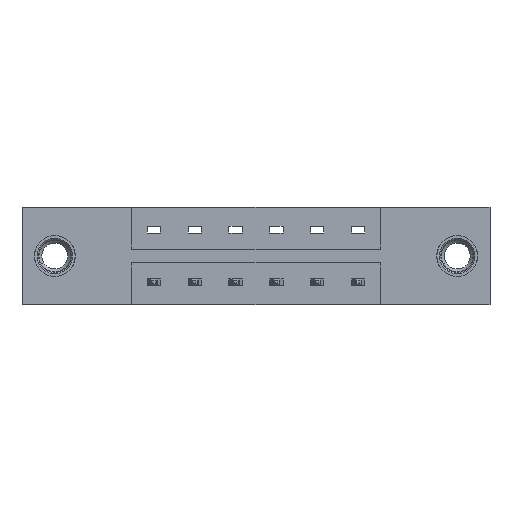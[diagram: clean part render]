
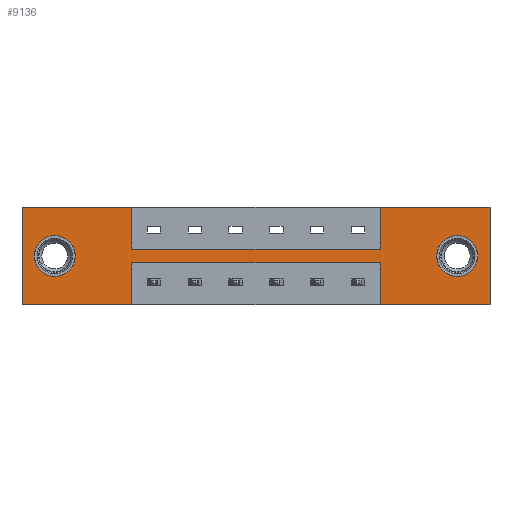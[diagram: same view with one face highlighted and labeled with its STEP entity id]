
A CAD part, front view. The second image highlights one B-rep face of the part: STEP entity #9136.
In plain terms, the highlighted planar face has unit normal (0, -1, 0).
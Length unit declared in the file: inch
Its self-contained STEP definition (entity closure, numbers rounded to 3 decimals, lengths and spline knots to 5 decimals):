
#42 = EDGE_CURVE ( 'NONE', #6262, #1896, #3276, .T. ) ;
#59 = CARTESIAN_POINT ( 'NONE',  ( 0.125, 0., -0.185 ) ) ;
#103 = DIRECTION ( 'NONE',  ( 0., 0., -1. ) ) ;
#153 = CARTESIAN_POINT ( 'NONE',  ( 0.4175, 0., -0.2115 ) ) ;
#176 = VECTOR ( 'NONE', #2613, 39.37008 ) ;
#224 = CIRCLE ( 'NONE', #9170, 0.078 ) ;
#268 = ORIENTED_EDGE ( 'NONE', *, *, #4116, .F. ) ;
#306 = EDGE_CURVE ( 'NONE', #5752, #7579, #224, .T. ) ;
#448 = EDGE_CURVE ( 'NONE', #5555, #4148, #8287, .T. ) ;
#486 = EDGE_CURVE ( 'NONE', #7261, #4726, #8028, .T. ) ;
#496 = CARTESIAN_POINT ( 'NONE',  ( 1.784, 0., -0.37 ) ) ;
#527 = VECTOR ( 'NONE', #1350, 39.37008 ) ;
#580 = EDGE_CURVE ( 'NONE', #7845, #5018, #1256, .T. ) ;
#640 = ORIENTED_EDGE ( 'NONE', *, *, #42, .F. ) ;
#680 = CARTESIAN_POINT ( 'NONE',  ( 0.125, 0., -0.107 ) ) ;
#698 = ORIENTED_EDGE ( 'NONE', *, *, #8571, .T. ) ;
#761 = DIRECTION ( 'NONE',  ( 0., 0., 1. ) ) ;
#824 = CARTESIAN_POINT ( 'NONE',  ( 0.4175, 0., -0.37 ) ) ;
#830 = ORIENTED_EDGE ( 'NONE', *, *, #5171, .T. ) ;
#857 = CARTESIAN_POINT ( 'NONE',  ( 0., 0., -0.37 ) ) ;
#1021 = LINE ( 'NONE', #7696, #5488 ) ;
#1100 = VERTEX_POINT ( 'NONE', #4235 ) ;
#1187 = ORIENTED_EDGE ( 'NONE', *, *, #1646, .F. ) ;
#1199 = FACE_BOUND ( 'NONE', #2375, .T. ) ;
#1221 = AXIS2_PLACEMENT_3D ( 'NONE', #6427, #3348, #5008 ) ;
#1256 = LINE ( 'NONE', #9368, #5358 ) ;
#1301 = VECTOR ( 'NONE', #6805, 39.37008 ) ;
#1348 = EDGE_CURVE ( 'NONE', #1100, #7279, #3021, .T. ) ;
#1350 = DIRECTION ( 'NONE',  ( 0., 0., -1. ) ) ;
#1412 = VECTOR ( 'NONE', #7191, 39.37008 ) ;
#1428 = CARTESIAN_POINT ( 'NONE',  ( 1.3665, 0., -0.2115 ) ) ;
#1646 = EDGE_CURVE ( 'NONE', #5018, #5555, #4294, .T. ) ;
#1680 = AXIS2_PLACEMENT_3D ( 'NONE', #6038, #4714, #5991 ) ;
#1739 = CARTESIAN_POINT ( 'NONE',  ( 1.659, 0., -0.263 ) ) ;
#1790 = DIRECTION ( 'NONE',  ( 0., 0., -1. ) ) ;
#1799 = CARTESIAN_POINT ( 'NONE',  ( 1.659, 0., -0.185 ) ) ;
#1852 = CARTESIAN_POINT ( 'NONE',  ( 1.3665, 0., 0. ) ) ;
#1877 = DIRECTION ( 'NONE',  ( -1., 0., 0. ) ) ;
#1897 = EDGE_CURVE ( 'NONE', #7939, #5543, #6997, .T. ) ;
#1896 = VERTEX_POINT ( 'NONE', #5483 ) ;
#2048 = AXIS2_PLACEMENT_3D ( 'NONE', #2392, #3271, #6209 ) ;
#2211 = ORIENTED_EDGE ( 'NONE', *, *, #2682, .F. ) ;
#2288 = DIRECTION ( 'NONE',  ( -1., 0., 0. ) ) ;
#2375 = EDGE_LOOP ( 'NONE', ( #2495, #830 ) ) ;
#2392 = CARTESIAN_POINT ( 'NONE',  ( 0.125, 0., -0.185 ) ) ;
#2489 = VERTEX_POINT ( 'NONE', #1852 ) ;
#2495 = ORIENTED_EDGE ( 'NONE', *, *, #306, .T. ) ;
#2613 = DIRECTION ( 'NONE',  ( 1., 0., 0. ) ) ;
#2682 = EDGE_CURVE ( 'NONE', #4148, #6349, #5589, .T. ) ;
#2778 = CIRCLE ( 'NONE', #1680, 0.078 ) ;
#2873 = CARTESIAN_POINT ( 'NONE',  ( 0., 0., -0.37 ) ) ;
#3009 = VECTOR ( 'NONE', #1877, 39.37008 ) ;
#3021 = CIRCLE ( 'NONE', #9168, 0.078 ) ;
#3271 = DIRECTION ( 'NONE',  ( 0., 1., 0. ) ) ;
#3276 = LINE ( 'NONE', #8254, #1301 ) ;
#3292 = CIRCLE ( 'NONE', #2048, 0.078 ) ;
#3348 = DIRECTION ( 'NONE',  ( 0., -1., 0. ) ) ;
#3495 = ORIENTED_EDGE ( 'NONE', *, *, #580, .F. ) ;
#3519 = EDGE_LOOP ( 'NONE', ( #9091, #698 ) ) ;
#3556 = CARTESIAN_POINT ( 'NONE',  ( 0.4175, 0., -0.2115 ) ) ;
#3586 = DIRECTION ( 'NONE',  ( 0., 0., 1. ) ) ;
#3748 = ORIENTED_EDGE ( 'NONE', *, *, #486, .F. ) ;
#3759 = CARTESIAN_POINT ( 'NONE',  ( 0., 0., 0. ) ) ;
#3983 = DIRECTION ( 'NONE',  ( 0., 0., -1. ) ) ;
#4116 = EDGE_CURVE ( 'NONE', #4726, #7845, #8816, .T. ) ;
#4148 = VERTEX_POINT ( 'NONE', #824 ) ;
#4235 = CARTESIAN_POINT ( 'NONE',  ( 1.659, 0., -0.107 ) ) ;
#4294 = LINE ( 'NONE', #3556, #1412 ) ;
#4295 = CARTESIAN_POINT ( 'NONE',  ( 1.784, 0., 0. ) ) ;
#4336 = LINE ( 'NONE', #8020, #6308 ) ;
#4349 = EDGE_CURVE ( 'NONE', #6349, #7939, #4384, .T. ) ;
#4384 = LINE ( 'NONE', #7871, #8032 ) ;
#4665 = CARTESIAN_POINT ( 'NONE',  ( 0.4175, 0., 0. ) ) ;
#4714 = DIRECTION ( 'NONE',  ( 0., 1., 0. ) ) ;
#4726 = VERTEX_POINT ( 'NONE', #496 ) ;
#4767 = EDGE_LOOP ( 'NONE', ( #3495, #268, #3748, #9145, #5228, #640, #7189, #6249, #6372, #2211, #5713, #1187 ) ) ;
#4962 = PLANE ( 'NONE',  #1221 ) ;
#5008 = DIRECTION ( 'NONE',  ( 0., 0., -1. ) ) ;
#5018 = VERTEX_POINT ( 'NONE', #1428 ) ;
#5033 = DIRECTION ( 'NONE',  ( 0., 1., 0. ) ) ;
#5156 = CARTESIAN_POINT ( 'NONE',  ( 0.125, 0., -0.263 ) ) ;
#5158 = EDGE_CURVE ( 'NONE', #5543, #6262, #6074, .T. ) ;
#5171 = EDGE_CURVE ( 'NONE', #7579, #5752, #3292, .T. ) ;
#5203 = VECTOR ( 'NONE', #103, 39.37008 ) ;
#5228 = ORIENTED_EDGE ( 'NONE', *, *, #9371, .F. ) ;
#5358 = VECTOR ( 'NONE', #9418, 39.37008 ) ;
#5483 = CARTESIAN_POINT ( 'NONE',  ( 1.3665, 0., -0.1585 ) ) ;
#5488 = VECTOR ( 'NONE', #8247, 39.37008 ) ;
#5543 = VERTEX_POINT ( 'NONE', #4665 ) ;
#5555 = VERTEX_POINT ( 'NONE', #153 ) ;
#5583 = FACE_BOUND ( 'NONE', #3519, .T. ) ;
#5589 = LINE ( 'NONE', #6240, #3009 ) ;
#5596 = EDGE_CURVE ( 'NONE', #2489, #7261, #1021, .T. ) ;
#5677 = CARTESIAN_POINT ( 'NONE',  ( 1.3665, 0., -0.37 ) ) ;
#5713 = ORIENTED_EDGE ( 'NONE', *, *, #448, .F. ) ;
#5752 = VERTEX_POINT ( 'NONE', #680 ) ;
#5991 = DIRECTION ( 'NONE',  ( 0., 0., -1. ) ) ;
#6038 = CARTESIAN_POINT ( 'NONE',  ( 1.659, 0., -0.185 ) ) ;
#6074 = LINE ( 'NONE', #6840, #7442 ) ;
#6200 = CARTESIAN_POINT ( 'NONE',  ( 1.784, 0., 0. ) ) ;
#6209 = DIRECTION ( 'NONE',  ( 0., 0., 1. ) ) ;
#6240 = CARTESIAN_POINT ( 'NONE',  ( 0., 0., -0.37 ) ) ;
#6249 = ORIENTED_EDGE ( 'NONE', *, *, #1897, .F. ) ;
#6262 = VERTEX_POINT ( 'NONE', #8809 ) ;
#6308 = VECTOR ( 'NONE', #761, 39.37008 ) ;
#6349 = VERTEX_POINT ( 'NONE', #857 ) ;
#6372 = ORIENTED_EDGE ( 'NONE', *, *, #4349, .F. ) ;
#6427 = CARTESIAN_POINT ( 'NONE',  ( 0., 0., -0.37 ) ) ;
#6805 = DIRECTION ( 'NONE',  ( 1., 0., 0. ) ) ;
#6840 = CARTESIAN_POINT ( 'NONE',  ( 0.4175, 0., -0.1585 ) ) ;
#6889 = DIRECTION ( 'NONE',  ( 0., 1., 0. ) ) ;
#6997 = LINE ( 'NONE', #9206, #176 ) ;
#7106 = FACE_OUTER_BOUND ( 'NONE', #4767, .T. ) ;
#7189 = ORIENTED_EDGE ( 'NONE', *, *, #5158, .F. ) ;
#7191 = DIRECTION ( 'NONE',  ( -1., 0., 0. ) ) ;
#7261 = VERTEX_POINT ( 'NONE', #6200 ) ;
#7279 = VERTEX_POINT ( 'NONE', #1739 ) ;
#7442 = VECTOR ( 'NONE', #1790, 39.37008 ) ;
#7579 = VERTEX_POINT ( 'NONE', #5156 ) ;
#7696 = CARTESIAN_POINT ( 'NONE',  ( 0., 0., 0. ) ) ;
#7845 = VERTEX_POINT ( 'NONE', #5677 ) ;
#7871 = CARTESIAN_POINT ( 'NONE',  ( 0., 0., 0. ) ) ;
#7939 = VERTEX_POINT ( 'NONE', #3759 ) ;
#8014 = DIRECTION ( 'NONE',  ( 0., 0., 1. ) ) ;
#8020 = CARTESIAN_POINT ( 'NONE',  ( 1.3665, 0., -0.1585 ) ) ;
#8028 = LINE ( 'NONE', #4295, #527 ) ;
#8032 = VECTOR ( 'NONE', #8014, 39.37008 ) ;
#8197 = CARTESIAN_POINT ( 'NONE',  ( 0.4175, 0., -0.2115 ) ) ;
#8247 = DIRECTION ( 'NONE',  ( 1., 0., 0. ) ) ;
#8254 = CARTESIAN_POINT ( 'NONE',  ( 0.4175, 0., -0.1585 ) ) ;
#8287 = LINE ( 'NONE', #8197, #5203 ) ;
#8571 = EDGE_CURVE ( 'NONE', #7279, #1100, #2778, .T. ) ;
#8809 = CARTESIAN_POINT ( 'NONE',  ( 0.4175, 0., -0.1585 ) ) ;
#8816 = LINE ( 'NONE', #2873, #9221 ) ;
#9091 = ORIENTED_EDGE ( 'NONE', *, *, #1348, .T. ) ;
#9136 = ADVANCED_FACE ( 'NONE', ( #5583, #1199, #7106 ), #4962, .T. ) ;
#9145 = ORIENTED_EDGE ( 'NONE', *, *, #5596, .F. ) ;
#9168 = AXIS2_PLACEMENT_3D ( 'NONE', #1799, #6889, #3983 ) ;
#9170 = AXIS2_PLACEMENT_3D ( 'NONE', #59, #5033, #3586 ) ;
#9206 = CARTESIAN_POINT ( 'NONE',  ( 0., 0., 0. ) ) ;
#9221 = VECTOR ( 'NONE', #2288, 39.37008 ) ;
#9368 = CARTESIAN_POINT ( 'NONE',  ( 1.3665, 0., -0.2115 ) ) ;
#9371 = EDGE_CURVE ( 'NONE', #1896, #2489, #4336, .T. ) ;
#9418 = DIRECTION ( 'NONE',  ( 0., 0., 1. ) ) ;
